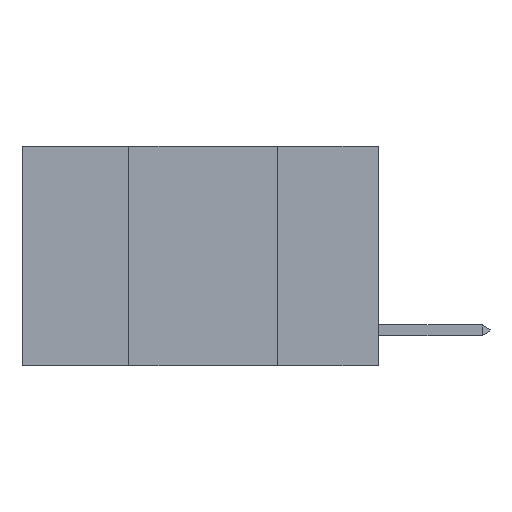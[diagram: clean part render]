
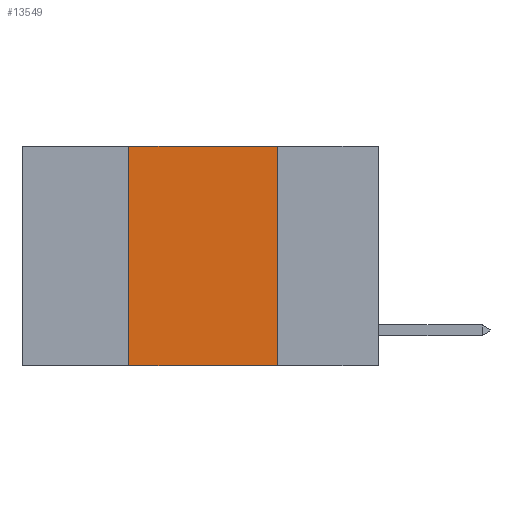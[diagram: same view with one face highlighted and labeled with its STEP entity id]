
A CAD part, left-side view. The second image highlights one B-rep face of the part: STEP entity #13549.
In plain terms, the highlighted planar face has unit normal (-1, 0, 0).
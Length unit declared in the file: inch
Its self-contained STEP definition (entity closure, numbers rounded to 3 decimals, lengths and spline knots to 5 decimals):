
#254 = EDGE_CURVE ( 'NONE', #3755, #1382, #10793, .T. ) ;
#1382 = VERTEX_POINT ( 'NONE', #17394 ) ;
#1693 = DIRECTION ( 'NONE',  ( 0., -1., 0. ) ) ;
#2831 = CARTESIAN_POINT ( 'NONE',  ( 0., 0.6, 0. ) ) ;
#3119 = CARTESIAN_POINT ( 'NONE',  ( 0., 0.6, -0.37 ) ) ;
#3315 = LINE ( 'NONE', #2831, #4272 ) ;
#3755 = VERTEX_POINT ( 'NONE', #11437 ) ;
#4064 = LINE ( 'NONE', #12251, #5741 ) ;
#4122 = PLANE ( 'NONE',  #7082 ) ;
#4272 = VECTOR ( 'NONE', #6133, 39.37008 ) ;
#4367 = EDGE_CURVE ( 'NONE', #6960, #1382, #17434, .T. ) ;
#5197 = EDGE_LOOP ( 'NONE', ( #10818, #5304, #12601, #6488 ) ) ;
#5294 = CARTESIAN_POINT ( 'NONE',  ( 0., 0.17, 0. ) ) ;
#5304 = ORIENTED_EDGE ( 'NONE', *, *, #15657, .F. ) ;
#5741 = VECTOR ( 'NONE', #12541, 39.37008 ) ;
#6133 = DIRECTION ( 'NONE',  ( 0., -1., 0. ) ) ;
#6488 = ORIENTED_EDGE ( 'NONE', *, *, #254, .T. ) ;
#6960 = VERTEX_POINT ( 'NONE', #5294 ) ;
#7072 = VECTOR ( 'NONE', #9194, 39.37008 ) ;
#7082 = AXIS2_PLACEMENT_3D ( 'NONE', #19410, #7103, #14724 ) ;
#7103 = DIRECTION ( 'NONE',  ( 1., 0., 0. ) ) ;
#9194 = DIRECTION ( 'NONE',  ( 0., 0., -1. ) ) ;
#9732 = EDGE_CURVE ( 'NONE', #3755, #14740, #4064, .T. ) ;
#10793 = LINE ( 'NONE', #3119, #15401 ) ;
#10818 = ORIENTED_EDGE ( 'NONE', *, *, #4367, .F. ) ;
#11437 = CARTESIAN_POINT ( 'NONE',  ( 0., 0.42, -0.37 ) ) ;
#12251 = CARTESIAN_POINT ( 'NONE',  ( 0., 0.42, 0. ) ) ;
#12541 = DIRECTION ( 'NONE',  ( 0., 0., 1. ) ) ;
#12601 = ORIENTED_EDGE ( 'NONE', *, *, #9732, .F. ) ;
#13187 = CARTESIAN_POINT ( 'NONE',  ( 0., 0.42, 0. ) ) ;
#13549 = ADVANCED_FACE ( 'NONE', ( #19643 ), #4122, .F. ) ;
#14724 = DIRECTION ( 'NONE',  ( 0., 0., -1. ) ) ;
#14740 = VERTEX_POINT ( 'NONE', #13187 ) ;
#15401 = VECTOR ( 'NONE', #1693, 39.37008 ) ;
#15657 = EDGE_CURVE ( 'NONE', #14740, #6960, #3315, .T. ) ;
#17394 = CARTESIAN_POINT ( 'NONE',  ( 0., 0.17, -0.37 ) ) ;
#17434 = LINE ( 'NONE', #19563, #7072 ) ;
#19410 = CARTESIAN_POINT ( 'NONE',  ( 0., 0.6, 0. ) ) ;
#19563 = CARTESIAN_POINT ( 'NONE',  ( 0., 0.17, 0. ) ) ;
#19643 = FACE_OUTER_BOUND ( 'NONE', #5197, .T. ) ;
